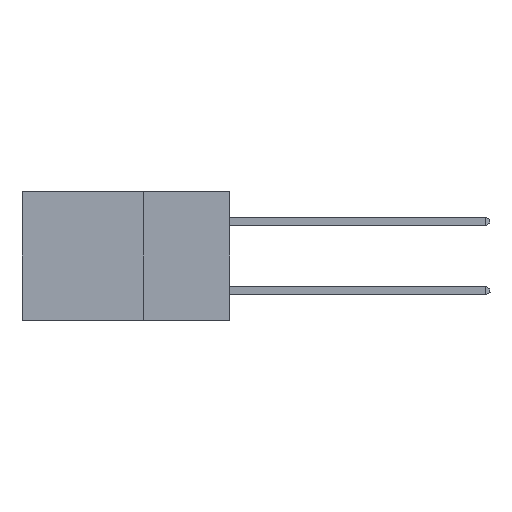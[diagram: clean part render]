
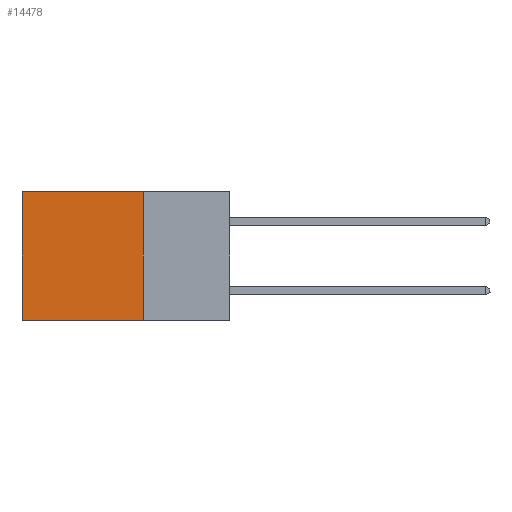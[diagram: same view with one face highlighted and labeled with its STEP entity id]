
A CAD part, left-side view. The second image highlights one B-rep face of the part: STEP entity #14478.
In plain terms, the highlighted planar face has unit normal (-1, 0, 0).
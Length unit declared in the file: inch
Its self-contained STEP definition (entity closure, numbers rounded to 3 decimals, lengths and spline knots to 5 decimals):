
#29 = CARTESIAN_POINT ( 'NONE',  ( 0.298, 0.25, -0.37 ) ) ;
#52 = DIRECTION ( 'NONE',  ( 1., 0., 0. ) ) ;
#547 = FACE_OUTER_BOUND ( 'NONE', #11892, .T. ) ;
#1457 = VERTEX_POINT ( 'NONE', #29 ) ;
#1831 = DIRECTION ( 'NONE',  ( 0., 0., -1. ) ) ;
#1986 = CARTESIAN_POINT ( 'NONE',  ( 0.298, 0.6, -0.37 ) ) ;
#2482 = VERTEX_POINT ( 'NONE', #12638 ) ;
#3782 = CARTESIAN_POINT ( 'NONE',  ( 0.298, 0.25, -0.37 ) ) ;
#5105 = ORIENTED_EDGE ( 'NONE', *, *, #6854, .T. ) ;
#6401 = ORIENTED_EDGE ( 'NONE', *, *, #9333, .F. ) ;
#6854 = EDGE_CURVE ( 'NONE', #2482, #19029, #9412, .T. ) ;
#8293 = AXIS2_PLACEMENT_3D ( 'NONE', #16696, #52, #15058 ) ;
#8682 = DIRECTION ( 'NONE',  ( 0., 1., 0. ) ) ;
#9333 = EDGE_CURVE ( 'NONE', #1457, #12870, #9608, .T. ) ;
#9412 = LINE ( 'NONE', #17430, #10728 ) ;
#9608 = LINE ( 'NONE', #3782, #12219 ) ;
#10007 = ORIENTED_EDGE ( 'NONE', *, *, #16808, .T. ) ;
#10728 = VECTOR ( 'NONE', #15942, 39.37008 ) ;
#11892 = EDGE_LOOP ( 'NONE', ( #10007, #6401, #15532, #5105 ) ) ;
#12219 = VECTOR ( 'NONE', #8682, 39.37008 ) ;
#12638 = CARTESIAN_POINT ( 'NONE',  ( 0.298, 0.25, 0. ) ) ;
#12870 = VERTEX_POINT ( 'NONE', #1986 ) ;
#14192 = EDGE_CURVE ( 'NONE', #2482, #1457, #16458, .T. ) ;
#14478 = ADVANCED_FACE ( 'NONE', ( #547 ), #19985, .F. ) ;
#15001 = CARTESIAN_POINT ( 'NONE',  ( 0.298, 0.6, 0. ) ) ;
#15058 = DIRECTION ( 'NONE',  ( 0., 0., -1. ) ) ;
#15532 = ORIENTED_EDGE ( 'NONE', *, *, #14192, .F. ) ;
#15942 = DIRECTION ( 'NONE',  ( 0., 1., 0. ) ) ;
#16458 = LINE ( 'NONE', #17558, #17795 ) ;
#16696 = CARTESIAN_POINT ( 'NONE',  ( 0.298, 0.25, 0. ) ) ;
#16808 = EDGE_CURVE ( 'NONE', #19029, #12870, #16899, .T. ) ;
#16899 = LINE ( 'NONE', #15001, #20308 ) ;
#17430 = CARTESIAN_POINT ( 'NONE',  ( 0.298, 0.25, 0. ) ) ;
#17485 = DIRECTION ( 'NONE',  ( 0., 0., -1. ) ) ;
#17558 = CARTESIAN_POINT ( 'NONE',  ( 0.298, 0.25, 0. ) ) ;
#17795 = VECTOR ( 'NONE', #17485, 39.37008 ) ;
#19029 = VERTEX_POINT ( 'NONE', #20954 ) ;
#19985 = PLANE ( 'NONE',  #8293 ) ;
#20308 = VECTOR ( 'NONE', #1831, 39.37008 ) ;
#20954 = CARTESIAN_POINT ( 'NONE',  ( 0.298, 0.6, 0. ) ) ;
